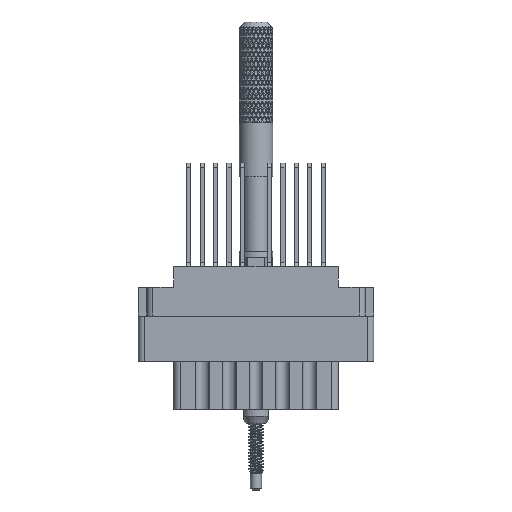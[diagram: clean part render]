
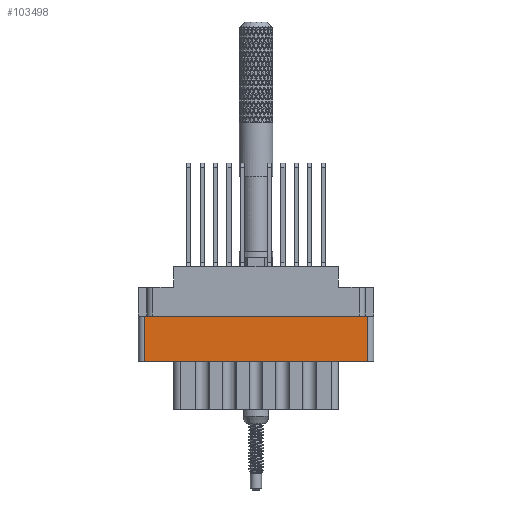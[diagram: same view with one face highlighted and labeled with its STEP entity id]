
A CAD part, front view. The second image highlights one B-rep face of the part: STEP entity #103498.
In plain terms, the highlighted planar face has unit normal (0, -1, 0).
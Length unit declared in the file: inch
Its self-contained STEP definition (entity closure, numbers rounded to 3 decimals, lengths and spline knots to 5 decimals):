
#606 = DIRECTION ( 'NONE',  ( 0., -1., 0. ) ) ;
#841 = DIRECTION ( 'NONE',  ( 1., 0., 0. ) ) ;
#1166 = EDGE_LOOP ( 'NONE', ( #183840, #115337, #135704, #121357 ) ) ;
#4496 = LINE ( 'NONE', #76859, #54255 ) ;
#21428 = VECTOR ( 'NONE', #841, 39.37008 ) ;
#22236 = FACE_OUTER_BOUND ( 'NONE', #1166, .T. ) ;
#23702 = VERTEX_POINT ( 'NONE', #186386 ) ;
#25004 = CARTESIAN_POINT ( 'NONE',  ( 0.624, -0.343, -0.798 ) ) ;
#27693 = EDGE_CURVE ( 'NONE', #164423, #23702, #4496, .T. ) ;
#31862 = CARTESIAN_POINT ( 'NONE',  ( 0., -0.343, -0.277 ) ) ;
#32585 = DIRECTION ( 'NONE',  ( -1., 0., 0. ) ) ;
#41321 = VECTOR ( 'NONE', #67947, 39.37008 ) ;
#44285 = CARTESIAN_POINT ( 'NONE',  ( -0.656, -0.343, -0.798 ) ) ;
#45383 = DIRECTION ( 'NONE',  ( 0., 0., -1. ) ) ;
#54255 = VECTOR ( 'NONE', #32585, 39.37008 ) ;
#54446 = EDGE_CURVE ( 'NONE', #71188, #105523, #148169, .T. ) ;
#57349 = CARTESIAN_POINT ( 'NONE',  ( 0.624, -0.343, -0.529 ) ) ;
#58802 = PLANE ( 'NONE',  #131080 ) ;
#67947 = DIRECTION ( 'NONE',  ( 0., 0., 1. ) ) ;
#71188 = VERTEX_POINT ( 'NONE', #158725 ) ;
#76859 = CARTESIAN_POINT ( 'NONE',  ( 0., -0.343, -0.529 ) ) ;
#78699 = VECTOR ( 'NONE', #45383, 39.37008 ) ;
#79817 = LINE ( 'NONE', #25004, #41321 ) ;
#81202 = CARTESIAN_POINT ( 'NONE',  ( 0.624, -0.343, -0.277 ) ) ;
#86106 = DIRECTION ( 'NONE',  ( 0., 0., -1. ) ) ;
#103498 = ADVANCED_FACE ( 'NONE', ( #22236 ), #58802, .T. ) ;
#103793 = EDGE_CURVE ( 'NONE', #71188, #23702, #158108, .T. ) ;
#105523 = VERTEX_POINT ( 'NONE', #81202 ) ;
#115337 = ORIENTED_EDGE ( 'NONE', *, *, #103793, .T. ) ;
#121357 = ORIENTED_EDGE ( 'NONE', *, *, #181420, .T. ) ;
#131080 = AXIS2_PLACEMENT_3D ( 'NONE', #44285, #606, #86106 ) ;
#135704 = ORIENTED_EDGE ( 'NONE', *, *, #27693, .F. ) ;
#148169 = LINE ( 'NONE', #31862, #21428 ) ;
#158108 = LINE ( 'NONE', #158794, #78699 ) ;
#158725 = CARTESIAN_POINT ( 'NONE',  ( -0.624, -0.343, -0.277 ) ) ;
#158794 = CARTESIAN_POINT ( 'NONE',  ( -0.624, -0.343, -0.798 ) ) ;
#164423 = VERTEX_POINT ( 'NONE', #57349 ) ;
#181420 = EDGE_CURVE ( 'NONE', #164423, #105523, #79817, .T. ) ;
#183840 = ORIENTED_EDGE ( 'NONE', *, *, #54446, .F. ) ;
#186386 = CARTESIAN_POINT ( 'NONE',  ( -0.624, -0.343, -0.529 ) ) ;
